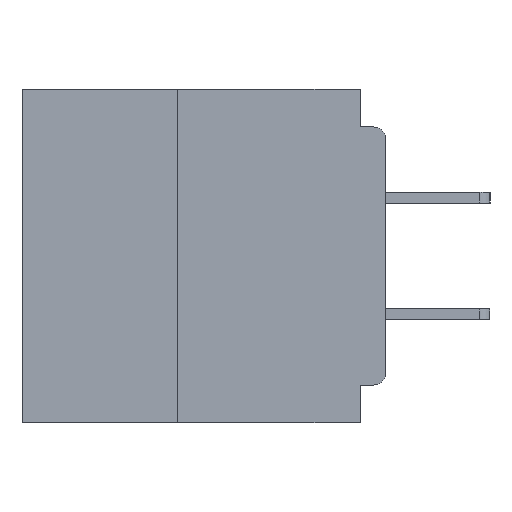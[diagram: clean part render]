
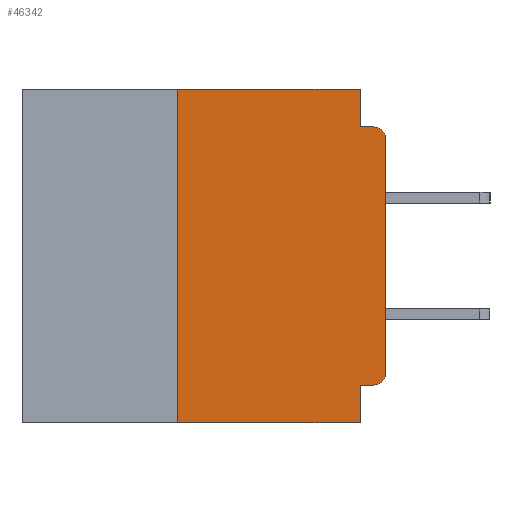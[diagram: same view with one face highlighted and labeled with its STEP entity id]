
A CAD part, left-side view. The second image highlights one B-rep face of the part: STEP entity #46342.
In plain terms, the highlighted planar face has unit normal (-1, 0, 0).
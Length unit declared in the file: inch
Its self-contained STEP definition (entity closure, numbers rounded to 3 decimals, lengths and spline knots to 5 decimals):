
#27 = CARTESIAN_POINT ( 'NONE',  ( 0., 0.437, -0.4 ) ) ;
#449 = CIRCLE ( 'NONE', #25334, 0.015 ) ;
#561 = CARTESIAN_POINT ( 'NONE',  ( 0., 0., -0.34 ) ) ;
#1008 = VECTOR ( 'NONE', #45206, 39.37008 ) ;
#2195 = LINE ( 'NONE', #16305, #1008 ) ;
#2719 = CARTESIAN_POINT ( 'NONE',  ( 0., 0.031, -0.4 ) ) ;
#2826 = VERTEX_POINT ( 'NONE', #35072 ) ;
#3124 = EDGE_CURVE ( 'NONE', #25203, #37354, #16078, .T. ) ;
#5172 = ORIENTED_EDGE ( 'NONE', *, *, #23913, .T. ) ;
#6469 = VECTOR ( 'NONE', #20332, 39.37008 ) ;
#6826 = ORIENTED_EDGE ( 'NONE', *, *, #15738, .F. ) ;
#7261 = LINE ( 'NONE', #36277, #33812 ) ;
#7375 = ORIENTED_EDGE ( 'NONE', *, *, #3124, .F. ) ;
#7411 = CARTESIAN_POINT ( 'NONE',  ( 0., 0.031, -0.355 ) ) ;
#8368 = VERTEX_POINT ( 'NONE', #27886 ) ;
#8861 = ORIENTED_EDGE ( 'NONE', *, *, #44316, .F. ) ;
#9047 = LINE ( 'NONE', #27, #25954 ) ;
#9234 = PLANE ( 'NONE',  #43526 ) ;
#9433 = LINE ( 'NONE', #11246, #46667 ) ;
#10627 = VECTOR ( 'NONE', #36083, 39.37008 ) ;
#11238 = CARTESIAN_POINT ( 'NONE',  ( 0., 0., 0. ) ) ;
#11246 = CARTESIAN_POINT ( 'NONE',  ( 0., 0.25, -0.4 ) ) ;
#11714 = VERTEX_POINT ( 'NONE', #43845 ) ;
#12044 = VECTOR ( 'NONE', #14838, 39.37008 ) ;
#12226 = CARTESIAN_POINT ( 'NONE',  ( 0., 0.015, -0.34 ) ) ;
#12885 = DIRECTION ( 'NONE',  ( 1., 0., 0. ) ) ;
#13082 = CARTESIAN_POINT ( 'NONE',  ( 0., 0.25, -0.4 ) ) ;
#13494 = AXIS2_PLACEMENT_3D ( 'NONE', #43101, #21438, #46671 ) ;
#14293 = CARTESIAN_POINT ( 'NONE',  ( 0., 0.031, -0.4 ) ) ;
#14838 = DIRECTION ( 'NONE',  ( 0., 0., 1. ) ) ;
#15738 = EDGE_CURVE ( 'NONE', #2826, #23010, #22142, .T. ) ;
#15823 = DIRECTION ( 'NONE',  ( 0., 0., -1. ) ) ;
#16018 = ORIENTED_EDGE ( 'NONE', *, *, #34216, .T. ) ;
#16046 = FACE_OUTER_BOUND ( 'NONE', #42667, .T. ) ;
#16078 = LINE ( 'NONE', #21222, #6469 ) ;
#16305 = CARTESIAN_POINT ( 'NONE',  ( 0., 0., -0.045 ) ) ;
#16353 = CARTESIAN_POINT ( 'NONE',  ( 0., 0.031, 0. ) ) ;
#16718 = EDGE_CURVE ( 'NONE', #42700, #23438, #9047, .T. ) ;
#16760 = ORIENTED_EDGE ( 'NONE', *, *, #39997, .F. ) ;
#17011 = VERTEX_POINT ( 'NONE', #23686 ) ;
#19179 = EDGE_CURVE ( 'NONE', #42700, #25203, #9433, .T. ) ;
#20332 = DIRECTION ( 'NONE',  ( 0., -1., 0. ) ) ;
#20439 = CARTESIAN_POINT ( 'NONE',  ( 0., 0.25, 0. ) ) ;
#21222 = CARTESIAN_POINT ( 'NONE',  ( 0., 0.437, 0. ) ) ;
#21438 = DIRECTION ( 'NONE',  ( -1., 0., 0. ) ) ;
#22142 = LINE ( 'NONE', #44648, #30615 ) ;
#22770 = LINE ( 'NONE', #11238, #12044 ) ;
#22919 = ORIENTED_EDGE ( 'NONE', *, *, #41014, .F. ) ;
#23010 = VERTEX_POINT ( 'NONE', #7411 ) ;
#23438 = VERTEX_POINT ( 'NONE', #2719 ) ;
#23686 = CARTESIAN_POINT ( 'NONE',  ( 0., 0.031, -0.045 ) ) ;
#23913 = EDGE_CURVE ( 'NONE', #2826, #43026, #449, .T. ) ;
#25203 = VERTEX_POINT ( 'NONE', #20439 ) ;
#25334 = AXIS2_PLACEMENT_3D ( 'NONE', #12226, #37481, #15823 ) ;
#25954 = VECTOR ( 'NONE', #43627, 39.37008 ) ;
#26806 = ORIENTED_EDGE ( 'NONE', *, *, #40911, .T. ) ;
#27040 = CARTESIAN_POINT ( 'NONE',  ( 0., 0.437, 0. ) ) ;
#27886 = CARTESIAN_POINT ( 'NONE',  ( 0., 0.015, -0.045 ) ) ;
#28012 = ORIENTED_EDGE ( 'NONE', *, *, #19179, .F. ) ;
#29880 = CIRCLE ( 'NONE', #13494, 0.015 ) ;
#30615 = VECTOR ( 'NONE', #41048, 39.37008 ) ;
#32855 = DIRECTION ( 'NONE',  ( 0., 0., 1. ) ) ;
#33812 = VECTOR ( 'NONE', #43734, 39.37008 ) ;
#34216 = EDGE_CURVE ( 'NONE', #43026, #11714, #22770, .T. ) ;
#35072 = CARTESIAN_POINT ( 'NONE',  ( 0., 0.015, -0.355 ) ) ;
#36083 = DIRECTION ( 'NONE',  ( 0., 0., -1. ) ) ;
#36277 = CARTESIAN_POINT ( 'NONE',  ( 0., 0.031, 0. ) ) ;
#37354 = VERTEX_POINT ( 'NONE', #16353 ) ;
#37481 = DIRECTION ( 'NONE',  ( -1., 0., 0. ) ) ;
#38144 = DIRECTION ( 'NONE',  ( 0., 0., -1. ) ) ;
#39452 = LINE ( 'NONE', #14293, #10627 ) ;
#39997 = EDGE_CURVE ( 'NONE', #17011, #8368, #2195, .T. ) ;
#40911 = EDGE_CURVE ( 'NONE', #11714, #8368, #29880, .T. ) ;
#41014 = EDGE_CURVE ( 'NONE', #37354, #17011, #7261, .T. ) ;
#41048 = DIRECTION ( 'NONE',  ( 0., 1., 0. ) ) ;
#42005 = ORIENTED_EDGE ( 'NONE', *, *, #16718, .T. ) ;
#42667 = EDGE_LOOP ( 'NONE', ( #16018, #26806, #16760, #22919, #7375, #28012, #42005, #8861, #6826, #5172 ) ) ;
#42700 = VERTEX_POINT ( 'NONE', #13082 ) ;
#43026 = VERTEX_POINT ( 'NONE', #561 ) ;
#43101 = CARTESIAN_POINT ( 'NONE',  ( 0., 0.015, -0.06 ) ) ;
#43526 = AXIS2_PLACEMENT_3D ( 'NONE', #27040, #12885, #38144 ) ;
#43627 = DIRECTION ( 'NONE',  ( 0., -1., 0. ) ) ;
#43734 = DIRECTION ( 'NONE',  ( 0., 0., -1. ) ) ;
#43845 = CARTESIAN_POINT ( 'NONE',  ( 0., 0., -0.06 ) ) ;
#44316 = EDGE_CURVE ( 'NONE', #23010, #23438, #39452, .T. ) ;
#44648 = CARTESIAN_POINT ( 'NONE',  ( 0., 0., -0.355 ) ) ;
#45206 = DIRECTION ( 'NONE',  ( 0., -1., 0. ) ) ;
#46342 = ADVANCED_FACE ( 'NONE', ( #16046 ), #9234, .F. ) ;
#46667 = VECTOR ( 'NONE', #32855, 39.37008 ) ;
#46671 = DIRECTION ( 'NONE',  ( 0., 0., -1. ) ) ;
